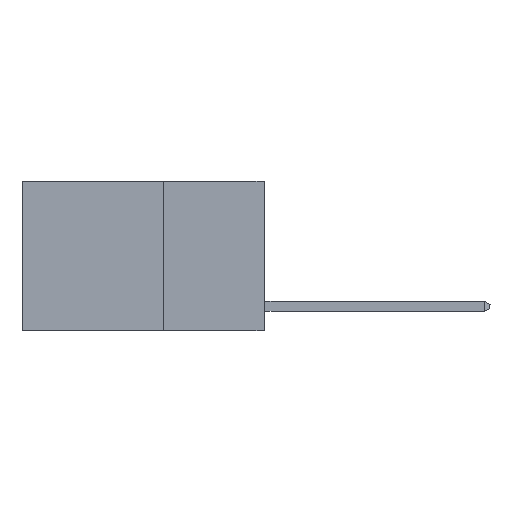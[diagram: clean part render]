
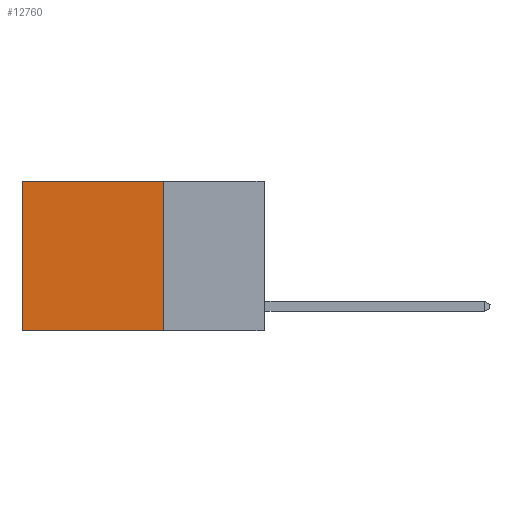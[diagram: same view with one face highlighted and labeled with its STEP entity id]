
A CAD part, left-side view. The second image highlights one B-rep face of the part: STEP entity #12760.
In plain terms, the highlighted planar face has unit normal (-1, 0, 0).
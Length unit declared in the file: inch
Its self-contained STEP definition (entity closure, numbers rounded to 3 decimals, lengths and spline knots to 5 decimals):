
#261 = ORIENTED_EDGE ( 'NONE', *, *, #9733, .F. ) ;
#1833 = VECTOR ( 'NONE', #8299, 39.37008 ) ;
#2108 = CARTESIAN_POINT ( 'NONE',  ( 0.2625, 0.6, 0. ) ) ;
#2612 = DIRECTION ( 'NONE',  ( 0., 0., -1. ) ) ;
#2829 = CARTESIAN_POINT ( 'NONE',  ( 0.2625, 0.25, 0. ) ) ;
#3375 = VERTEX_POINT ( 'NONE', #4754 ) ;
#3579 = EDGE_LOOP ( 'NONE', ( #4410, #261, #13724, #3924 ) ) ;
#3776 = EDGE_CURVE ( 'NONE', #11821, #4836, #19082, .T. ) ;
#3924 = ORIENTED_EDGE ( 'NONE', *, *, #10861, .T. ) ;
#4249 = LINE ( 'NONE', #4400, #8382 ) ;
#4392 = DIRECTION ( 'NONE',  ( 0., 0., -1. ) ) ;
#4400 = CARTESIAN_POINT ( 'NONE',  ( 0.2625, 0.25, 0. ) ) ;
#4410 = ORIENTED_EDGE ( 'NONE', *, *, #19141, .T. ) ;
#4754 = CARTESIAN_POINT ( 'NONE',  ( 0.2625, 0.6, 0. ) ) ;
#4836 = VERTEX_POINT ( 'NONE', #16047 ) ;
#5045 = LINE ( 'NONE', #12419, #16700 ) ;
#5291 = AXIS2_PLACEMENT_3D ( 'NONE', #2829, #13562, #4392 ) ;
#5405 = CARTESIAN_POINT ( 'NONE',  ( 0.2625, 0.25, 0. ) ) ;
#5914 = PLANE ( 'NONE',  #5291 ) ;
#8299 = DIRECTION ( 'NONE',  ( 0., 0., -1. ) ) ;
#8382 = VECTOR ( 'NONE', #15111, 39.37008 ) ;
#8967 = VERTEX_POINT ( 'NONE', #11162 ) ;
#9134 = LINE ( 'NONE', #2108, #1833 ) ;
#9473 = DIRECTION ( 'NONE',  ( 0., 1., 0. ) ) ;
#9733 = EDGE_CURVE ( 'NONE', #4836, #8967, #5045, .T. ) ;
#10861 = EDGE_CURVE ( 'NONE', #11821, #3375, #4249, .T. ) ;
#11162 = CARTESIAN_POINT ( 'NONE',  ( 0.2625, 0.6, -0.37 ) ) ;
#11821 = VERTEX_POINT ( 'NONE', #5405 ) ;
#11846 = CARTESIAN_POINT ( 'NONE',  ( 0.2625, 0.25, 0. ) ) ;
#12419 = CARTESIAN_POINT ( 'NONE',  ( 0.2625, 0.25, -0.37 ) ) ;
#12760 = ADVANCED_FACE ( 'NONE', ( #16706 ), #5914, .F. ) ;
#13562 = DIRECTION ( 'NONE',  ( 1., 0., 0. ) ) ;
#13724 = ORIENTED_EDGE ( 'NONE', *, *, #3776, .F. ) ;
#14677 = VECTOR ( 'NONE', #2612, 39.37008 ) ;
#15111 = DIRECTION ( 'NONE',  ( 0., 1., 0. ) ) ;
#16047 = CARTESIAN_POINT ( 'NONE',  ( 0.2625, 0.25, -0.37 ) ) ;
#16700 = VECTOR ( 'NONE', #9473, 39.37008 ) ;
#16706 = FACE_OUTER_BOUND ( 'NONE', #3579, .T. ) ;
#19082 = LINE ( 'NONE', #11846, #14677 ) ;
#19141 = EDGE_CURVE ( 'NONE', #3375, #8967, #9134, .T. ) ;
